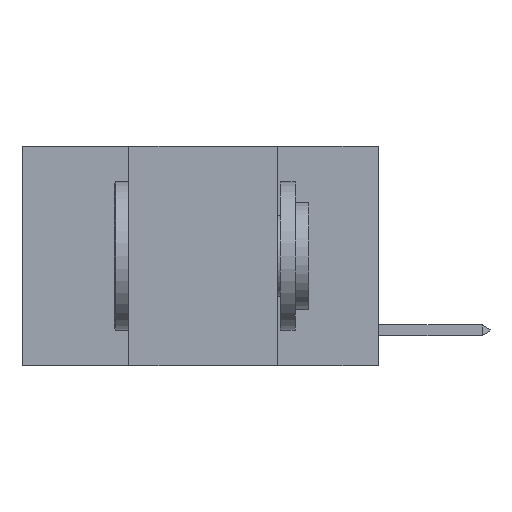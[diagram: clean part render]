
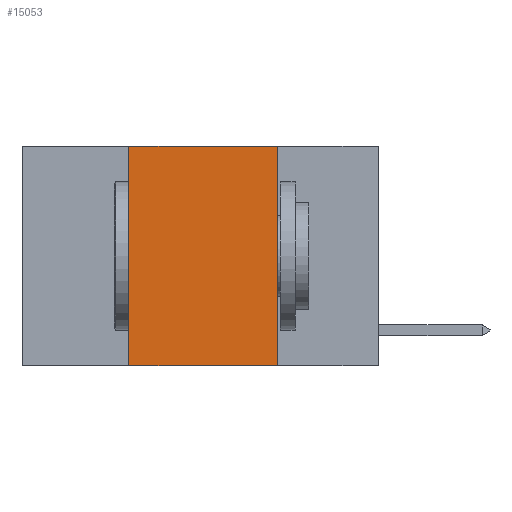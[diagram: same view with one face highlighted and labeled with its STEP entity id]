
A CAD part, left-side view. The second image highlights one B-rep face of the part: STEP entity #15053.
In plain terms, the highlighted planar face has unit normal (-1, 0, 0).
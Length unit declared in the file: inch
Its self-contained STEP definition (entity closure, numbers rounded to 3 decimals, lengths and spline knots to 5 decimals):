
#39 = CARTESIAN_POINT ( 'NONE',  ( 0., 0.42, 0. ) ) ;
#56 = LINE ( 'NONE', #6931, #16986 ) ;
#645 = CARTESIAN_POINT ( 'NONE',  ( 0., 0.17, -0.37 ) ) ;
#936 = VERTEX_POINT ( 'NONE', #645 ) ;
#956 = ORIENTED_EDGE ( 'NONE', *, *, #10727, .T. ) ;
#1393 = PLANE ( 'NONE',  #14069 ) ;
#1465 = CARTESIAN_POINT ( 'NONE',  ( 0., 0.6, 0. ) ) ;
#2151 = ORIENTED_EDGE ( 'NONE', *, *, #20562, .F. ) ;
#2631 = VERTEX_POINT ( 'NONE', #39 ) ;
#2919 = DIRECTION ( 'NONE',  ( 0., 0., -1. ) ) ;
#3115 = DIRECTION ( 'NONE',  ( 0., 0., -1. ) ) ;
#3308 = ORIENTED_EDGE ( 'NONE', *, *, #9625, .F. ) ;
#3672 = EDGE_LOOP ( 'NONE', ( #2151, #4613, #3308, #956 ) ) ;
#4218 = VERTEX_POINT ( 'NONE', #14036 ) ;
#4613 = ORIENTED_EDGE ( 'NONE', *, *, #14230, .F. ) ;
#6199 = VERTEX_POINT ( 'NONE', #13825 ) ;
#6597 = DIRECTION ( 'NONE',  ( 0., -1., 0. ) ) ;
#6931 = CARTESIAN_POINT ( 'NONE',  ( 0., 0.42, 0. ) ) ;
#6992 = LINE ( 'NONE', #19601, #14167 ) ;
#9625 = EDGE_CURVE ( 'NONE', #6199, #2631, #56, .T. ) ;
#10727 = EDGE_CURVE ( 'NONE', #6199, #936, #6992, .T. ) ;
#10774 = VECTOR ( 'NONE', #13546, 39.37008 ) ;
#11243 = FACE_OUTER_BOUND ( 'NONE', #3672, .T. ) ;
#11858 = VECTOR ( 'NONE', #2919, 39.37008 ) ;
#12362 = LINE ( 'NONE', #17561, #11858 ) ;
#12964 = DIRECTION ( 'NONE',  ( 1., 0., 0. ) ) ;
#13546 = DIRECTION ( 'NONE',  ( 0., -1., 0. ) ) ;
#13825 = CARTESIAN_POINT ( 'NONE',  ( 0., 0.42, -0.37 ) ) ;
#14036 = CARTESIAN_POINT ( 'NONE',  ( 0., 0.17, 0. ) ) ;
#14069 = AXIS2_PLACEMENT_3D ( 'NONE', #1465, #12964, #3115 ) ;
#14167 = VECTOR ( 'NONE', #6597, 39.37008 ) ;
#14230 = EDGE_CURVE ( 'NONE', #2631, #4218, #19864, .T. ) ;
#15053 = ADVANCED_FACE ( 'NONE', ( #11243 ), #1393, .F. ) ;
#16762 = DIRECTION ( 'NONE',  ( 0., 0., 1. ) ) ;
#16986 = VECTOR ( 'NONE', #16762, 39.37008 ) ;
#17561 = CARTESIAN_POINT ( 'NONE',  ( 0., 0.17, 0. ) ) ;
#18310 = CARTESIAN_POINT ( 'NONE',  ( 0., 0.6, 0. ) ) ;
#19601 = CARTESIAN_POINT ( 'NONE',  ( 0., 0.6, -0.37 ) ) ;
#19864 = LINE ( 'NONE', #18310, #10774 ) ;
#20562 = EDGE_CURVE ( 'NONE', #4218, #936, #12362, .T. ) ;
